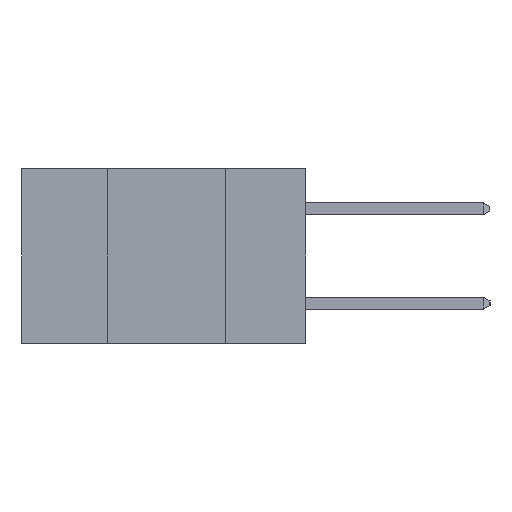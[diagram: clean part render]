
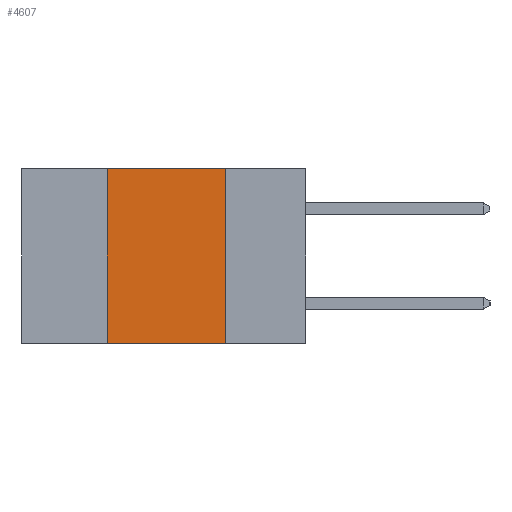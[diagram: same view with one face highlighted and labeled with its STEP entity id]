
A CAD part, left-side view. The second image highlights one B-rep face of the part: STEP entity #4607.
In plain terms, the highlighted planar face has unit normal (-1, 0, 0).
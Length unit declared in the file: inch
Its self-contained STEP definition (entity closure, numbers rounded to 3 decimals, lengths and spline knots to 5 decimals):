
#38 = CARTESIAN_POINT ( 'NONE',  ( 0., 0.42, -0.37 ) ) ;
#437 = VERTEX_POINT ( 'NONE', #1768 ) ;
#1683 = DIRECTION ( 'NONE',  ( 0., -1., 0. ) ) ;
#1694 = CARTESIAN_POINT ( 'NONE',  ( 0., 0.6, -0.37 ) ) ;
#1768 = CARTESIAN_POINT ( 'NONE',  ( 0., 0.42, -0.37 ) ) ;
#2016 = ORIENTED_EDGE ( 'NONE', *, *, #7736, .F. ) ;
#2059 = CARTESIAN_POINT ( 'NONE',  ( 0., 0.17, 0. ) ) ;
#2297 = ORIENTED_EDGE ( 'NONE', *, *, #4552, .F. ) ;
#2956 = LINE ( 'NONE', #38, #7373 ) ;
#3332 = DIRECTION ( 'NONE',  ( 0., 0., -1. ) ) ;
#3497 = CARTESIAN_POINT ( 'NONE',  ( 0., 0.42, 0. ) ) ;
#3654 = DIRECTION ( 'NONE',  ( 1., 0., 0. ) ) ;
#3845 = CARTESIAN_POINT ( 'NONE',  ( 0., 0.6, 0. ) ) ;
#3948 = VECTOR ( 'NONE', #6344, 39.37008 ) ;
#4187 = VECTOR ( 'NONE', #1683, 39.37008 ) ;
#4497 = PLANE ( 'NONE',  #8424 ) ;
#4552 = EDGE_CURVE ( 'NONE', #437, #9049, #2956, .T. ) ;
#4567 = VERTEX_POINT ( 'NONE', #8150 ) ;
#4607 = ADVANCED_FACE ( 'NONE', ( #6832 ), #4497, .F. ) ;
#4619 = VERTEX_POINT ( 'NONE', #2059 ) ;
#4634 = ORIENTED_EDGE ( 'NONE', *, *, #8633, .T. ) ;
#5969 = EDGE_CURVE ( 'NONE', #4619, #4567, #10766, .T. ) ;
#6344 = DIRECTION ( 'NONE',  ( 0., -1., 0. ) ) ;
#6353 = CARTESIAN_POINT ( 'NONE',  ( 0., 0.6, 0. ) ) ;
#6832 = FACE_OUTER_BOUND ( 'NONE', #9582, .T. ) ;
#7373 = VECTOR ( 'NONE', #11143, 39.37008 ) ;
#7736 = EDGE_CURVE ( 'NONE', #9049, #4619, #8870, .T. ) ;
#8150 = CARTESIAN_POINT ( 'NONE',  ( 0., 0.17, -0.37 ) ) ;
#8285 = VECTOR ( 'NONE', #10103, 39.37008 ) ;
#8424 = AXIS2_PLACEMENT_3D ( 'NONE', #3845, #3654, #3332 ) ;
#8633 = EDGE_CURVE ( 'NONE', #437, #4567, #10285, .T. ) ;
#8870 = LINE ( 'NONE', #6353, #3948 ) ;
#9049 = VERTEX_POINT ( 'NONE', #3497 ) ;
#9582 = EDGE_LOOP ( 'NONE', ( #10968, #2016, #2297, #4634 ) ) ;
#10089 = CARTESIAN_POINT ( 'NONE',  ( 0., 0.17, -0.37 ) ) ;
#10103 = DIRECTION ( 'NONE',  ( 0., 0., -1. ) ) ;
#10285 = LINE ( 'NONE', #1694, #4187 ) ;
#10766 = LINE ( 'NONE', #10089, #8285 ) ;
#10968 = ORIENTED_EDGE ( 'NONE', *, *, #5969, .F. ) ;
#11143 = DIRECTION ( 'NONE',  ( 0., 0., 1. ) ) ;
